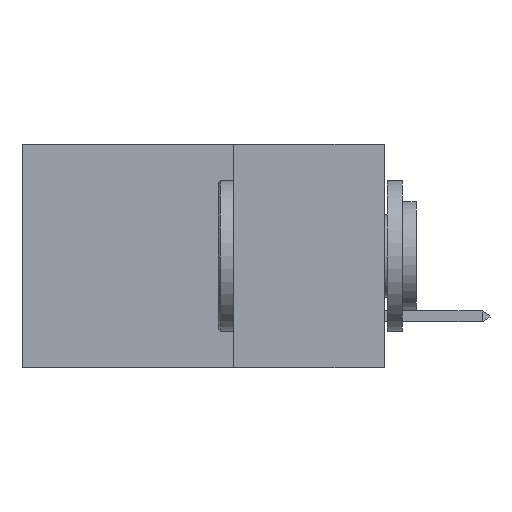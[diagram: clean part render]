
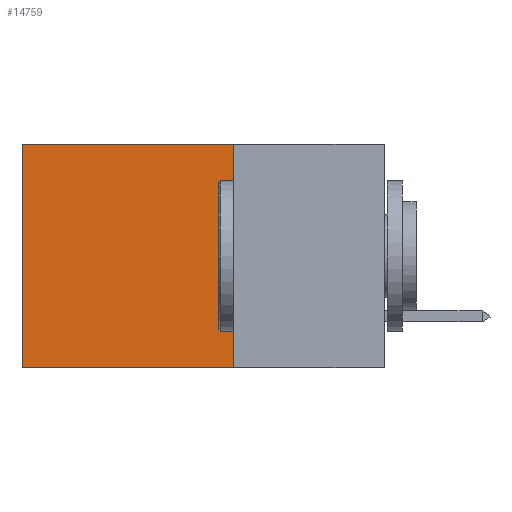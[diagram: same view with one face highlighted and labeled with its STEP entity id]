
A CAD part, left-side view. The second image highlights one B-rep face of the part: STEP entity #14759.
In plain terms, the highlighted planar face has unit normal (-1, 0, 0).
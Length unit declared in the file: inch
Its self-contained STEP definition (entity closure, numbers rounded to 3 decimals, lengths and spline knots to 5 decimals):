
#338 = CARTESIAN_POINT ( 'NONE',  ( 0.2875, 0.25, 0. ) ) ;
#429 = VECTOR ( 'NONE', #2813, 39.37008 ) ;
#501 = PLANE ( 'NONE',  #12305 ) ;
#1748 = DIRECTION ( 'NONE',  ( 1., 0., 0. ) ) ;
#2032 = LINE ( 'NONE', #11210, #4857 ) ;
#2813 = DIRECTION ( 'NONE',  ( 0., 0., -1. ) ) ;
#3335 = EDGE_CURVE ( 'NONE', #7121, #4494, #12572, .T. ) ;
#3424 = ORIENTED_EDGE ( 'NONE', *, *, #13959, .F. ) ;
#3680 = LINE ( 'NONE', #7627, #429 ) ;
#3994 = VECTOR ( 'NONE', #13650, 39.37008 ) ;
#4148 = EDGE_LOOP ( 'NONE', ( #10396, #3424, #11947, #10818 ) ) ;
#4494 = VERTEX_POINT ( 'NONE', #5753 ) ;
#4857 = VECTOR ( 'NONE', #10318, 39.37008 ) ;
#5753 = CARTESIAN_POINT ( 'NONE',  ( 0.2875, 0.6, 0. ) ) ;
#6664 = FACE_OUTER_BOUND ( 'NONE', #4148, .T. ) ;
#7121 = VERTEX_POINT ( 'NONE', #338 ) ;
#7124 = EDGE_CURVE ( 'NONE', #4494, #9293, #3680, .T. ) ;
#7541 = CARTESIAN_POINT ( 'NONE',  ( 0.2875, 0.25, -0.37 ) ) ;
#7627 = CARTESIAN_POINT ( 'NONE',  ( 0.2875, 0.6, 0. ) ) ;
#9073 = CARTESIAN_POINT ( 'NONE',  ( 0.2875, 0.25, 0. ) ) ;
#9293 = VERTEX_POINT ( 'NONE', #14870 ) ;
#9323 = EDGE_CURVE ( 'NONE', #7121, #9529, #2032, .T. ) ;
#9529 = VERTEX_POINT ( 'NONE', #10814 ) ;
#9530 = CARTESIAN_POINT ( 'NONE',  ( 0.2875, 0.25, 0. ) ) ;
#10285 = DIRECTION ( 'NONE',  ( 0., 0., -1. ) ) ;
#10318 = DIRECTION ( 'NONE',  ( 0., 0., -1. ) ) ;
#10396 = ORIENTED_EDGE ( 'NONE', *, *, #7124, .T. ) ;
#10474 = LINE ( 'NONE', #7541, #3994 ) ;
#10736 = DIRECTION ( 'NONE',  ( 0., 1., 0. ) ) ;
#10814 = CARTESIAN_POINT ( 'NONE',  ( 0.2875, 0.25, -0.37 ) ) ;
#10818 = ORIENTED_EDGE ( 'NONE', *, *, #3335, .T. ) ;
#11210 = CARTESIAN_POINT ( 'NONE',  ( 0.2875, 0.25, 0. ) ) ;
#11947 = ORIENTED_EDGE ( 'NONE', *, *, #9323, .F. ) ;
#12194 = VECTOR ( 'NONE', #10736, 39.37008 ) ;
#12305 = AXIS2_PLACEMENT_3D ( 'NONE', #9073, #1748, #10285 ) ;
#12572 = LINE ( 'NONE', #9530, #12194 ) ;
#13650 = DIRECTION ( 'NONE',  ( 0., 1., 0. ) ) ;
#13959 = EDGE_CURVE ( 'NONE', #9529, #9293, #10474, .T. ) ;
#14759 = ADVANCED_FACE ( 'NONE', ( #6664 ), #501, .F. ) ;
#14870 = CARTESIAN_POINT ( 'NONE',  ( 0.2875, 0.6, -0.37 ) ) ;
